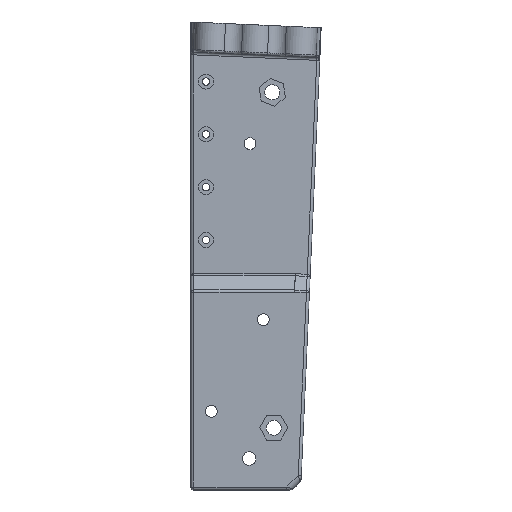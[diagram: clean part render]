
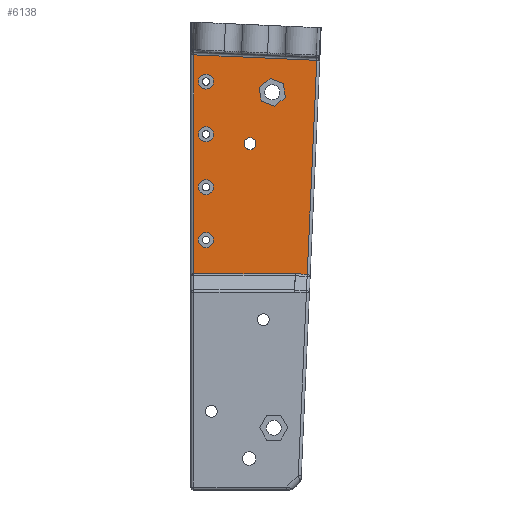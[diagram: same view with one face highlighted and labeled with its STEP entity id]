
A CAD part, left-side view. The second image highlights one B-rep face of the part: STEP entity #6138.
In plain terms, the highlighted planar face has unit normal (-1, 0, 0).
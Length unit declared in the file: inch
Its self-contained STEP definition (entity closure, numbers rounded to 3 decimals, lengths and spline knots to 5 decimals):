
#230=FACE_BOUND('',#1191,.T.);
#231=FACE_BOUND('',#1192,.T.);
#232=FACE_BOUND('',#1193,.T.);
#233=FACE_BOUND('',#1194,.T.);
#234=FACE_BOUND('',#1195,.T.);
#235=FACE_BOUND('',#1196,.T.);
#310=ELLIPSE('',#6680,0.11141,0.07874);
#516=CIRCLE('',#6656,0.1);
#517=CIRCLE('',#6657,0.1);
#521=CIRCLE('',#6663,0.1);
#522=CIRCLE('',#6664,0.1);
#526=CIRCLE('',#6670,0.1);
#527=CIRCLE('',#6671,0.1);
#531=CIRCLE('',#6677,0.1);
#532=CIRCLE('',#6678,0.1);
#533=CIRCLE('',#6681,0.07874);
#534=CIRCLE('',#6682,0.07874);
#808=FACE_OUTER_BOUND('',#1190,.T.);
#1190=EDGE_LOOP('',(#4881,#4882,#4883,#4884,#4885,#4886));
#1191=EDGE_LOOP('',(#4887,#4888));
#1192=EDGE_LOOP('',(#4889,#4890));
#1193=EDGE_LOOP('',(#4891,#4892));
#1194=EDGE_LOOP('',(#4893,#4894));
#1195=EDGE_LOOP('',(#4895,#4896,#4897,#4898,#4899,#4900));
#1196=EDGE_LOOP('',(#4901,#4902));
#1768=LINE('',#10493,#2297);
#1773=LINE('',#10558,#2302);
#1774=LINE('',#10562,#2303);
#1775=LINE('',#10563,#2304);
#1776=LINE('',#10564,#2305);
#1777=LINE('',#10571,#2306);
#1778=LINE('',#10573,#2307);
#1779=LINE('',#10575,#2308);
#1780=LINE('',#10577,#2309);
#1781=LINE('',#10579,#2310);
#1782=LINE('',#10580,#2311);
#2297=VECTOR('',#7899,0.3937);
#2302=VECTOR('',#7968,0.3937);
#2303=VECTOR('',#7971,0.3937);
#2304=VECTOR('',#7972,0.3937);
#2305=VECTOR('',#7973,0.3937);
#2306=VECTOR('',#7978,0.3937);
#2307=VECTOR('',#7979,0.3937);
#2308=VECTOR('',#7980,0.3937);
#2309=VECTOR('',#7981,0.3937);
#2310=VECTOR('',#7982,0.3937);
#2311=VECTOR('',#7983,0.3937);
#2878=VERTEX_POINT('',#10491);
#2879=VERTEX_POINT('',#10492);
#2885=VERTEX_POINT('',#10511);
#2886=VERTEX_POINT('',#10513);
#2890=VERTEX_POINT('',#10524);
#2891=VERTEX_POINT('',#10526);
#2895=VERTEX_POINT('',#10537);
#2896=VERTEX_POINT('',#10539);
#2900=VERTEX_POINT('',#10550);
#2901=VERTEX_POINT('',#10552);
#2902=VERTEX_POINT('',#10556);
#2903=VERTEX_POINT('',#10557);
#2904=VERTEX_POINT('',#10559);
#2905=VERTEX_POINT('',#10561);
#2906=VERTEX_POINT('',#10565);
#2907=VERTEX_POINT('',#10566);
#2908=VERTEX_POINT('',#10569);
#2909=VERTEX_POINT('',#10570);
#2910=VERTEX_POINT('',#10572);
#2911=VERTEX_POINT('',#10574);
#2912=VERTEX_POINT('',#10576);
#2913=VERTEX_POINT('',#10578);
#3607=EDGE_CURVE('',#2878,#2879,#1768,.T.);
#3616=EDGE_CURVE('',#2886,#2885,#516,.T.);
#3617=EDGE_CURVE('',#2885,#2886,#517,.T.);
#3622=EDGE_CURVE('',#2891,#2890,#521,.T.);
#3623=EDGE_CURVE('',#2890,#2891,#522,.T.);
#3628=EDGE_CURVE('',#2896,#2895,#526,.T.);
#3629=EDGE_CURVE('',#2895,#2896,#527,.T.);
#3634=EDGE_CURVE('',#2901,#2900,#531,.T.);
#3635=EDGE_CURVE('',#2900,#2901,#532,.T.);
#3636=EDGE_CURVE('',#2902,#2903,#1773,.T.);
#3637=EDGE_CURVE('',#2904,#2902,#310,.T.);
#3638=EDGE_CURVE('',#2905,#2904,#1774,.T.);
#3639=EDGE_CURVE('',#2879,#2905,#1775,.T.);
#3640=EDGE_CURVE('',#2903,#2878,#1776,.T.);
#3641=EDGE_CURVE('',#2906,#2907,#533,.T.);
#3642=EDGE_CURVE('',#2907,#2906,#534,.T.);
#3643=EDGE_CURVE('',#2908,#2909,#1777,.T.);
#3644=EDGE_CURVE('',#2909,#2910,#1778,.T.);
#3645=EDGE_CURVE('',#2910,#2911,#1779,.T.);
#3646=EDGE_CURVE('',#2911,#2912,#1780,.T.);
#3647=EDGE_CURVE('',#2912,#2913,#1781,.T.);
#3648=EDGE_CURVE('',#2913,#2908,#1782,.T.);
#4881=ORIENTED_EDGE('',*,*,#3636,.F.);
#4882=ORIENTED_EDGE('',*,*,#3637,.F.);
#4883=ORIENTED_EDGE('',*,*,#3638,.F.);
#4884=ORIENTED_EDGE('',*,*,#3639,.F.);
#4885=ORIENTED_EDGE('',*,*,#3607,.F.);
#4886=ORIENTED_EDGE('',*,*,#3640,.F.);
#4887=ORIENTED_EDGE('',*,*,#3634,.T.);
#4888=ORIENTED_EDGE('',*,*,#3635,.T.);
#4889=ORIENTED_EDGE('',*,*,#3628,.T.);
#4890=ORIENTED_EDGE('',*,*,#3629,.T.);
#4891=ORIENTED_EDGE('',*,*,#3622,.T.);
#4892=ORIENTED_EDGE('',*,*,#3623,.T.);
#4893=ORIENTED_EDGE('',*,*,#3641,.T.);
#4894=ORIENTED_EDGE('',*,*,#3642,.T.);
#4895=ORIENTED_EDGE('',*,*,#3643,.T.);
#4896=ORIENTED_EDGE('',*,*,#3644,.T.);
#4897=ORIENTED_EDGE('',*,*,#3645,.T.);
#4898=ORIENTED_EDGE('',*,*,#3646,.T.);
#4899=ORIENTED_EDGE('',*,*,#3647,.T.);
#4900=ORIENTED_EDGE('',*,*,#3648,.T.);
#4901=ORIENTED_EDGE('',*,*,#3616,.T.);
#4902=ORIENTED_EDGE('',*,*,#3617,.T.);
#5913=PLANE('',#6679);
#6138=ADVANCED_FACE('',(#808,#230,#231,#232,#233,#234,#235),#5913,.F.);
#6656=AXIS2_PLACEMENT_3D('',#10514,#7917,#7918);
#6657=AXIS2_PLACEMENT_3D('',#10515,#7919,#7920);
#6663=AXIS2_PLACEMENT_3D('',#10527,#7932,#7933);
#6664=AXIS2_PLACEMENT_3D('',#10528,#7934,#7935);
#6670=AXIS2_PLACEMENT_3D('',#10540,#7947,#7948);
#6671=AXIS2_PLACEMENT_3D('',#10541,#7949,#7950);
#6677=AXIS2_PLACEMENT_3D('',#10553,#7962,#7963);
#6678=AXIS2_PLACEMENT_3D('',#10554,#7964,#7965);
#6679=AXIS2_PLACEMENT_3D('',#10555,#7966,#7967);
#6680=AXIS2_PLACEMENT_3D('',#10560,#7969,#7970);
#6681=AXIS2_PLACEMENT_3D('',#10567,#7974,#7975);
#6682=AXIS2_PLACEMENT_3D('',#10568,#7976,#7977);
#7899=DIRECTION('',(0.,-0.999,-0.044));
#7917=DIRECTION('center_axis',(1.,0.,0.));
#7918=DIRECTION('ref_axis',(0.,0.,-1.));
#7919=DIRECTION('center_axis',(1.,0.,0.));
#7920=DIRECTION('ref_axis',(0.,0.,-1.));
#7932=DIRECTION('center_axis',(1.,0.,0.));
#7933=DIRECTION('ref_axis',(0.,0.,-1.));
#7934=DIRECTION('center_axis',(1.,0.,0.));
#7935=DIRECTION('ref_axis',(0.,0.,-1.));
#7947=DIRECTION('center_axis',(1.,0.,0.));
#7948=DIRECTION('ref_axis',(0.,0.,-1.));
#7949=DIRECTION('center_axis',(1.,0.,0.));
#7950=DIRECTION('ref_axis',(0.,0.,-1.));
#7962=DIRECTION('center_axis',(1.,0.,0.));
#7963=DIRECTION('ref_axis',(0.,0.,-1.));
#7964=DIRECTION('center_axis',(1.,0.,0.));
#7965=DIRECTION('ref_axis',(0.,0.,-1.));
#7966=DIRECTION('center_axis',(1.,0.,0.));
#7967=DIRECTION('ref_axis',(0.,0.,-1.));
#7968=DIRECTION('',(0.,1.,0.));
#7969=DIRECTION('center_axis',(-1.,0.,0.));
#7970=DIRECTION('ref_axis',(0.,-0.044,0.999));
#7971=DIRECTION('',(0.,0.999,0.044));
#7972=DIRECTION('',(0.,0.044,-0.999));
#7973=DIRECTION('',(0.,0.,1.));
#7974=DIRECTION('center_axis',(1.,0.,0.));
#7975=DIRECTION('ref_axis',(0.,0.,1.));
#7976=DIRECTION('center_axis',(1.,0.,0.));
#7977=DIRECTION('ref_axis',(0.,0.,1.));
#7978=DIRECTION('',(0.,0.153,0.988));
#7979=DIRECTION('',(0.,-0.78,0.626));
#7980=DIRECTION('',(0.,-0.932,-0.362));
#7981=DIRECTION('',(0.,-0.153,-0.988));
#7982=DIRECTION('',(0.,0.78,-0.626));
#7983=DIRECTION('',(0.,0.932,0.362));
#10491=CARTESIAN_POINT('',(-1.06693,-0.04275,5.79277));
#10492=CARTESIAN_POINT('',(-1.06693,-1.67223,5.7202));
#10493=CARTESIAN_POINT('',(-1.06693,-0.88771,5.75514));
#10511=CARTESIAN_POINT('',(-1.06693,-0.20416,5.53881));
#10513=CARTESIAN_POINT('',(-1.06693,-0.20416,5.33881));
#10514=CARTESIAN_POINT('Origin',(-1.06693,-0.20416,5.43881));
#10515=CARTESIAN_POINT('Origin',(-1.06693,-0.20416,5.43881));
#10524=CARTESIAN_POINT('',(-1.06693,-0.20416,4.83881));
#10526=CARTESIAN_POINT('',(-1.06693,-0.20416,4.63881));
#10527=CARTESIAN_POINT('Origin',(-1.06693,-0.20416,4.73881));
#10528=CARTESIAN_POINT('Origin',(-1.06693,-0.20416,4.73881));
#10537=CARTESIAN_POINT('',(-1.06693,-0.20416,4.13881));
#10539=CARTESIAN_POINT('',(-1.06693,-0.20416,3.93881));
#10540=CARTESIAN_POINT('Origin',(-1.06693,-0.20416,4.03881));
#10541=CARTESIAN_POINT('Origin',(-1.06693,-0.20416,4.03881));
#10550=CARTESIAN_POINT('',(-1.06693,-0.20416,3.43881));
#10552=CARTESIAN_POINT('',(-1.06693,-0.20416,3.23881));
#10553=CARTESIAN_POINT('Origin',(-1.06693,-0.20416,3.33881));
#10554=CARTESIAN_POINT('Origin',(-1.06693,-0.20416,3.33881));
#10555=CARTESIAN_POINT('Origin',(-1.06693,-0.8671,4.39551));
#10556=CARTESIAN_POINT('',(-1.06693,-1.38678,2.89196));
#10557=CARTESIAN_POINT('',(-1.06693,-0.04275,2.89196));
#10558=CARTESIAN_POINT('',(-1.06693,-0.4344,2.89196));
#10559=CARTESIAN_POINT('',(-1.06693,-1.38925,2.89191));
#10560=CARTESIAN_POINT('Origin',(-1.06693,-1.3843,2.78061));
#10561=CARTESIAN_POINT('',(-1.06693,-1.54596,2.88493));
#10562=CARTESIAN_POINT('',(-1.06693,-1.09497,2.90501));
#10563=CARTESIAN_POINT('',(-1.06693,-1.56451,3.30156));
#10564=CARTESIAN_POINT('',(-1.06693,-0.04275,2.19775));
#10565=CARTESIAN_POINT('',(-1.06693,-0.7874,4.53543));
#10566=CARTESIAN_POINT('',(-1.06693,-0.7874,4.69291));
#10567=CARTESIAN_POINT('Origin',(-1.06693,-0.7874,4.61417));
#10568=CARTESIAN_POINT('Origin',(-1.06693,-0.7874,4.61417));
#10569=CARTESIAN_POINT('',(-1.06693,-0.93739,5.17852));
#10570=CARTESIAN_POINT('',(-1.06693,-0.90892,5.36273));
#10571=CARTESIAN_POINT('',(-1.06693,-0.99565,4.80145));
#10572=CARTESIAN_POINT('',(-1.06693,-1.05421,5.47948));
#10573=CARTESIAN_POINT('',(-1.06693,-0.66008,5.16277));
#10574=CARTESIAN_POINT('',(-1.06693,-1.22797,5.41203));
#10575=CARTESIAN_POINT('',(-1.06693,-1.15575,5.44006));
#10576=CARTESIAN_POINT('',(-1.06693,-1.25643,5.22782));
#10577=CARTESIAN_POINT('',(-1.06693,-1.30047,4.94285));
#10578=CARTESIAN_POINT('',(-1.06693,-1.11114,5.11107));
#10579=CARTESIAN_POINT('',(-1.06693,-0.93495,4.96949));
#10580=CARTESIAN_POINT('',(-1.06693,-1.1258,5.10538));
